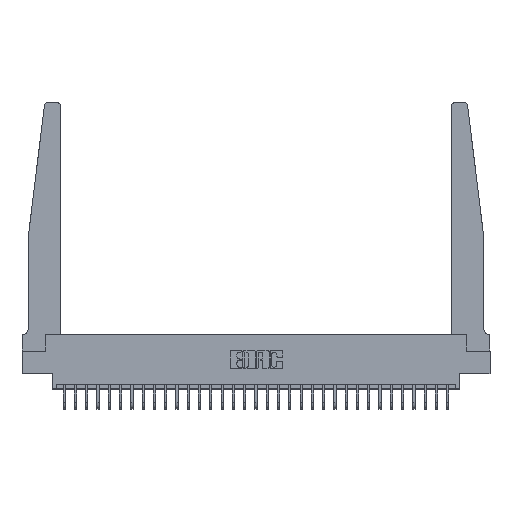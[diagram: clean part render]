
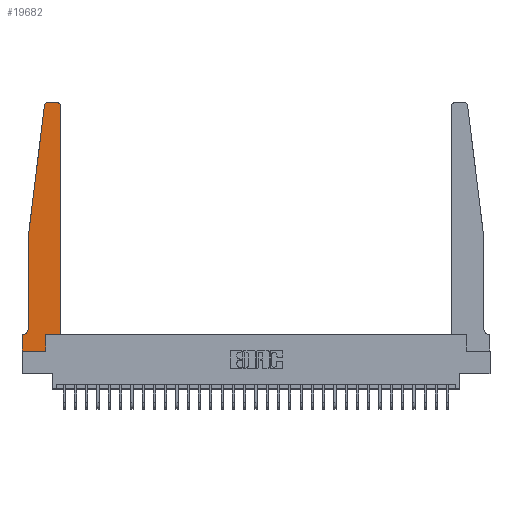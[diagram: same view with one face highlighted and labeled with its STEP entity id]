
A CAD part, top view. The second image highlights one B-rep face of the part: STEP entity #19682.
In plain terms, the highlighted planar face has unit normal (0, 0, 1).
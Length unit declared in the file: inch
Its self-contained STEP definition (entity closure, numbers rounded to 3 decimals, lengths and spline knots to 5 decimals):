
#298 = CIRCLE ( 'NONE', #10535, 0.03 ) ;
#324 = LINE ( 'NONE', #22130, #28326 ) ;
#771 = CARTESIAN_POINT ( 'NONE',  ( 0.425, 0.18, 0.37 ) ) ;
#1101 = LINE ( 'NONE', #27915, #15487 ) ;
#1224 = CARTESIAN_POINT ( 'NONE',  ( 0.25, 2.75, 0.37 ) ) ;
#1301 = DIRECTION ( 'NONE',  ( 0., 0., 1. ) ) ;
#1416 = CARTESIAN_POINT ( 'NONE',  ( 0., 0.1875, 0.37 ) ) ;
#1753 = VERTEX_POINT ( 'NONE', #15312 ) ;
#2359 = ORIENTED_EDGE ( 'NONE', *, *, #19834, .T. ) ;
#2650 = CIRCLE ( 'NONE', #16465, 0.05 ) ;
#3100 = EDGE_CURVE ( 'NONE', #1753, #20702, #22110, .T. ) ;
#3781 = VECTOR ( 'NONE', #15458, 39.37008 ) ;
#5034 = VERTEX_POINT ( 'NONE', #23128 ) ;
#5248 = DIRECTION ( 'NONE',  ( 0., 0., -1. ) ) ;
#5911 = ORIENTED_EDGE ( 'NONE', *, *, #23988, .T. ) ;
#6685 = ORIENTED_EDGE ( 'NONE', *, *, #28018, .T. ) ;
#6808 = CIRCLE ( 'NONE', #28014, 0.03 ) ;
#6861 = ORIENTED_EDGE ( 'NONE', *, *, #17132, .T. ) ;
#7392 = EDGE_CURVE ( 'NONE', #13894, #5034, #19963, .T. ) ;
#7542 = CARTESIAN_POINT ( 'NONE',  ( 0.065, 1.25, 0.37 ) ) ;
#7623 = VECTOR ( 'NONE', #27456, 39.37008 ) ;
#8112 = FACE_OUTER_BOUND ( 'NONE', #21039, .T. ) ;
#8318 = ORIENTED_EDGE ( 'NONE', *, *, #17307, .T. ) ;
#8720 = VERTEX_POINT ( 'NONE', #7542 ) ;
#8970 = VERTEX_POINT ( 'NONE', #18142 ) ;
#8994 = DIRECTION ( 'NONE',  ( 1., 0., 0. ) ) ;
#9027 = VERTEX_POINT ( 'NONE', #30285 ) ;
#9521 = LINE ( 'NONE', #17558, #21653 ) ;
#9524 = EDGE_CURVE ( 'NONE', #8720, #28496, #324, .T. ) ;
#10422 = PLANE ( 'NONE',  #18098 ) ;
#10535 = AXIS2_PLACEMENT_3D ( 'NONE', #18803, #20958, #18999 ) ;
#10574 = EDGE_CURVE ( 'NONE', #20702, #23192, #24596, .T. ) ;
#10778 = LINE ( 'NONE', #27071, #29885 ) ;
#12127 = DIRECTION ( 'NONE',  ( -0.122, -0.992, 0. ) ) ;
#12737 = DIRECTION ( 'NONE',  ( 0., -1., 0. ) ) ;
#13484 = EDGE_CURVE ( 'NONE', #22874, #24930, #17956, .T. ) ;
#13675 = CARTESIAN_POINT ( 'NONE',  ( 0.065, 0.2375, 0.37 ) ) ;
#13698 = ORIENTED_EDGE ( 'NONE', *, *, #9524, .T. ) ;
#13894 = VERTEX_POINT ( 'NONE', #24171 ) ;
#13898 = LINE ( 'NONE', #26230, #20114 ) ;
#14729 = DIRECTION ( 'NONE',  ( 0., -1., 0. ) ) ;
#14756 = VECTOR ( 'NONE', #22982, 39.37008 ) ;
#15312 = CARTESIAN_POINT ( 'NONE',  ( 0.2605, 0.18, 0.37 ) ) ;
#15458 = DIRECTION ( 'NONE',  ( -1., 0., 0. ) ) ;
#15487 = VECTOR ( 'NONE', #8994, 39.37008 ) ;
#15495 = ORIENTED_EDGE ( 'NONE', *, *, #10574, .T. ) ;
#15508 = ORIENTED_EDGE ( 'NONE', *, *, #13484, .T. ) ;
#16465 = AXIS2_PLACEMENT_3D ( 'NONE', #17178, #5248, #21701 ) ;
#16469 = CARTESIAN_POINT ( 'NONE',  ( 0.27653, 2.72, 0.37 ) ) ;
#17132 = EDGE_CURVE ( 'NONE', #28496, #22874, #2650, .T. ) ;
#17178 = CARTESIAN_POINT ( 'NONE',  ( 0.015, 0.2375, 0.37 ) ) ;
#17307 = EDGE_CURVE ( 'NONE', #8970, #1753, #10778, .T. ) ;
#17558 = CARTESIAN_POINT ( 'NONE',  ( 0., 0., 0.37 ) ) ;
#17644 = ORIENTED_EDGE ( 'NONE', *, *, #3100, .T. ) ;
#17789 = CARTESIAN_POINT ( 'NONE',  ( 0.065, 0.1875, 0.37 ) ) ;
#17956 = LINE ( 'NONE', #17789, #7623 ) ;
#18098 = AXIS2_PLACEMENT_3D ( 'NONE', #24472, #1301, #21988 ) ;
#18142 = CARTESIAN_POINT ( 'NONE',  ( 0.2605, 0., 0.37 ) ) ;
#18742 = DIRECTION ( 'NONE',  ( 0., 0., 1. ) ) ;
#18803 = CARTESIAN_POINT ( 'NONE',  ( 0.395, 2.72, 0.37 ) ) ;
#18999 = DIRECTION ( 'NONE',  ( 1., 0., 0. ) ) ;
#19050 = VECTOR ( 'NONE', #26051, 39.37008 ) ;
#19276 = CARTESIAN_POINT ( 'NONE',  ( 0.015, 0.1875, 0.37 ) ) ;
#19682 = ADVANCED_FACE ( 'NONE', ( #8112 ), #10422, .T. ) ;
#19834 = EDGE_CURVE ( 'NONE', #21828, #8970, #1101, .T. ) ;
#19963 = LINE ( 'NONE', #1224, #3781 ) ;
#20114 = VECTOR ( 'NONE', #12127, 39.37008 ) ;
#20702 = VERTEX_POINT ( 'NONE', #771 ) ;
#20819 = EDGE_CURVE ( 'NONE', #24930, #21828, #9521, .T. ) ;
#20958 = DIRECTION ( 'NONE',  ( 0., 0., 1. ) ) ;
#21039 = EDGE_LOOP ( 'NONE', ( #24786, #5911, #6685, #13698, #6861, #15508, #25839, #2359, #8318, #17644, #15495, #22928 ) ) ;
#21653 = VECTOR ( 'NONE', #12737, 39.37008 ) ;
#21701 = DIRECTION ( 'NONE',  ( -1., 0., 0. ) ) ;
#21828 = VERTEX_POINT ( 'NONE', #22443 ) ;
#21988 = DIRECTION ( 'NONE',  ( 1., 0., 0. ) ) ;
#22110 = LINE ( 'NONE', #29862, #14756 ) ;
#22130 = CARTESIAN_POINT ( 'NONE',  ( 0.065, 1.25, 0.37 ) ) ;
#22443 = CARTESIAN_POINT ( 'NONE',  ( 0., 0., 0.37 ) ) ;
#22874 = VERTEX_POINT ( 'NONE', #19276 ) ;
#22928 = ORIENTED_EDGE ( 'NONE', *, *, #26929, .T. ) ;
#22982 = DIRECTION ( 'NONE',  ( 1., 0., 0. ) ) ;
#23128 = CARTESIAN_POINT ( 'NONE',  ( 0.27653, 2.75, 0.37 ) ) ;
#23192 = VERTEX_POINT ( 'NONE', #23360 ) ;
#23360 = CARTESIAN_POINT ( 'NONE',  ( 0.425, 2.72, 0.37 ) ) ;
#23778 = CARTESIAN_POINT ( 'NONE',  ( 0.425, 0.18, 0.37 ) ) ;
#23988 = EDGE_CURVE ( 'NONE', #5034, #9027, #6808, .T. ) ;
#24171 = CARTESIAN_POINT ( 'NONE',  ( 0.395, 2.75, 0.37 ) ) ;
#24472 = CARTESIAN_POINT ( 'NONE',  ( 0., 0.1875, 0.37 ) ) ;
#24596 = LINE ( 'NONE', #23778, #19050 ) ;
#24786 = ORIENTED_EDGE ( 'NONE', *, *, #7392, .T. ) ;
#24930 = VERTEX_POINT ( 'NONE', #1416 ) ;
#25839 = ORIENTED_EDGE ( 'NONE', *, *, #20819, .T. ) ;
#26051 = DIRECTION ( 'NONE',  ( 0., 1., 0. ) ) ;
#26230 = CARTESIAN_POINT ( 'NONE',  ( 0.065, 1.25, 0.37 ) ) ;
#26750 = DIRECTION ( 'NONE',  ( 0., 1., 0. ) ) ;
#26929 = EDGE_CURVE ( 'NONE', #23192, #13894, #298, .T. ) ;
#27071 = CARTESIAN_POINT ( 'NONE',  ( 0.2605, 0.18, 0.37 ) ) ;
#27456 = DIRECTION ( 'NONE',  ( -1., 0., 0. ) ) ;
#27915 = CARTESIAN_POINT ( 'NONE',  ( 0., 0., 0.37 ) ) ;
#28014 = AXIS2_PLACEMENT_3D ( 'NONE', #16469, #18742, #28202 ) ;
#28018 = EDGE_CURVE ( 'NONE', #9027, #8720, #13898, .T. ) ;
#28202 = DIRECTION ( 'NONE',  ( 1., 0., 0. ) ) ;
#28326 = VECTOR ( 'NONE', #14729, 39.37008 ) ;
#28496 = VERTEX_POINT ( 'NONE', #13675 ) ;
#29862 = CARTESIAN_POINT ( 'NONE',  ( 0.425, 0.18, 0.37 ) ) ;
#29885 = VECTOR ( 'NONE', #26750, 39.37008 ) ;
#30285 = CARTESIAN_POINT ( 'NONE',  ( 0.24675, 2.72367, 0.37 ) ) ;
